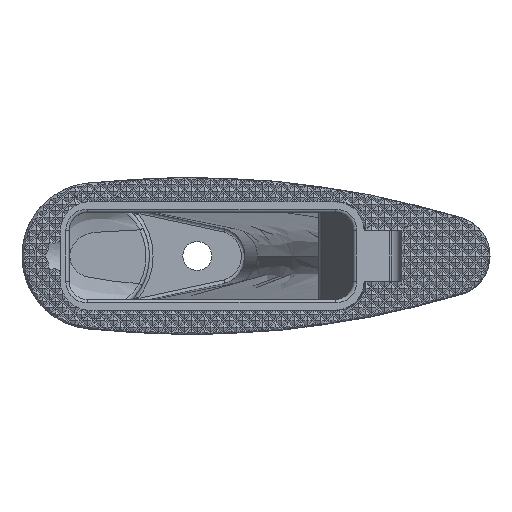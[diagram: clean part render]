
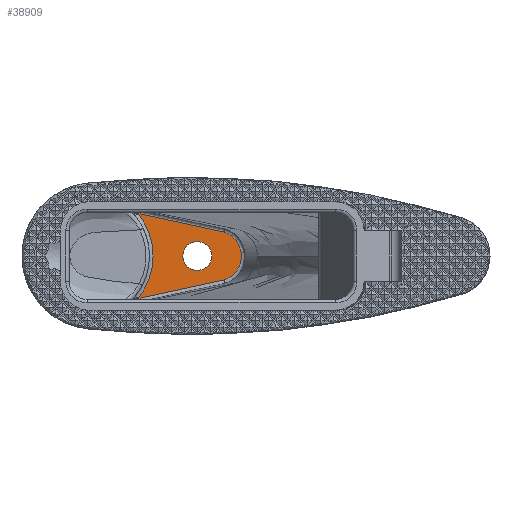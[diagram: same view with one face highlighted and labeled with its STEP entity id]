
A CAD part, left-side view. The second image highlights one B-rep face of the part: STEP entity #38909.
In plain terms, the highlighted planar face has unit normal (-1, 0, 0).
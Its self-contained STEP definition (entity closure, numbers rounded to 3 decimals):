
#926 = CIRCLE ( 'NONE', #54261, 4. ) ;
#2425 = FACE_BOUND ( 'NONE', #10219, .T. ) ;
#3760 = CARTESIAN_POINT ( 'NONE',  ( -210.6, -15.971, 6.591 ) ) ;
#4138 = CARTESIAN_POINT ( 'NONE',  ( -210.6, -20.515, 1.795 ) ) ;
#4658 = CARTESIAN_POINT ( 'NONE',  ( -210.6, 7.884, 11.758 ) ) ;
#5381 = VERTEX_POINT ( 'NONE', #7635 ) ;
#6216 = EDGE_CURVE ( 'NONE', #59459, #5381, #926, .T. ) ;
#7563 = B_SPLINE_CURVE_WITH_KNOTS ( 'NONE', 3,
 ( #16736, #67531, #17802, #61028, #34142, #17455, #34846 ),
 .UNSPECIFIED., .F., .F.,
 ( 4, 3, 4 ),
 ( 0., 0.011, 0.024 ),
 .UNSPECIFIED. ) ;
#7635 = CARTESIAN_POINT ( 'NONE',  ( -210.6, -8.516, 4. ) ) ;
#8342 = EDGE_CURVE ( 'NONE', #41749, #38159, #14809, .T. ) ;
#8493 = CARTESIAN_POINT ( 'NONE',  ( -210.6, -17.299, -6.008 ) ) ;
#9565 = CARTESIAN_POINT ( 'NONE',  ( -210.6, -20.74, 0.364 ) ) ;
#9740 = CARTESIAN_POINT ( 'NONE',  ( -210.6, 1.039, 10.275 ) ) ;
#9785 = CIRCLE ( 'NONE', #38876, 4. ) ;
#10219 = EDGE_LOOP ( 'NONE', ( #63972, #31793 ) ) ;
#11646 = ORIENTED_EDGE ( 'NONE', *, *, #71557, .T. ) ;
#12875 = CARTESIAN_POINT ( 'NONE',  ( -210.6, -16.648, -6.341 ) ) ;
#12945 = CARTESIAN_POINT ( 'NONE',  ( -210.6, -8.516, 0. ) ) ;
#13239 = CARTESIAN_POINT ( 'NONE',  ( -210.6, -16.314, -6.479 ) ) ;
#14061 = DIRECTION ( 'NONE',  ( -1., 0., 0. ) ) ;
#14809 = B_SPLINE_CURVE_WITH_KNOTS ( 'NONE', 3,
 ( #64927, #15202, #59492, #65276, #9740, #59859, #4658 ),
 .UNSPECIFIED., .F., .F.,
 ( 4, 3, 4 ),
 ( 0., 0.014, 0.024 ),
 .UNSPECIFIED. ) ;
#15202 = CARTESIAN_POINT ( 'NONE',  ( -210.6, -11.442, 7.573 ) ) ;
#15753 = CARTESIAN_POINT ( 'NONE',  ( -210.6, -20.599, -1.442 ) ) ;
#15930 = EDGE_LOOP ( 'NONE', ( #23929, #38214, #65621, #11646 ) ) ;
#16736 = CARTESIAN_POINT ( 'NONE',  ( -210.6, 7.884, -11.758 ) ) ;
#17455 = CARTESIAN_POINT ( 'NONE',  ( -210.6, -11.442, -7.573 ) ) ;
#17802 = CARTESIAN_POINT ( 'NONE',  ( -210.6, 1.039, -10.275 ) ) ;
#19174 = EDGE_CURVE ( 'NONE', #5381, #59459, #9785, .T. ) ;
#20528 = CARTESIAN_POINT ( 'NONE',  ( -210.6, -15.971, 6.591 ) ) ;
#21126 = DIRECTION ( 'NONE',  ( 1., 0., 0. ) ) ;
#23216 = CARTESIAN_POINT ( 'NONE',  ( -210.6, -15.971, -6.591 ) ) ;
#23788 = CARTESIAN_POINT ( 'NONE',  ( -210.6, -18.191, -5.392 ) ) ;
#23929 = ORIENTED_EDGE ( 'NONE', *, *, #8342, .T. ) ;
#24179 = DIRECTION ( 'NONE',  ( 0., 0., 1. ) ) ;
#25938 = CARTESIAN_POINT ( 'NONE',  ( -210.6, -18.49, 5.173 ) ) ;
#26308 = CARTESIAN_POINT ( 'NONE',  ( -210.6, -19.215, -4.361 ) ) ;
#26653 = CARTESIAN_POINT ( 'NONE',  ( -210.6, -20.74, -0.36 ) ) ;
#29328 = PLANE ( 'NONE',  #47952 ) ;
#29367 = VERTEX_POINT ( 'NONE', #23216 ) ;
#30736 = CARTESIAN_POINT ( 'NONE',  ( -210.6, -8.516, -4. ) ) ;
#31034 = CARTESIAN_POINT ( 'NONE',  ( -210.6, -20.292, 2.486 ) ) ;
#31381 = CARTESIAN_POINT ( 'NONE',  ( -210.6, -20.6, 1.437 ) ) ;
#31699 = AXIS2_PLACEMENT_3D ( 'NONE', #41950, #68092, #24179 ) ;
#31793 = ORIENTED_EDGE ( 'NONE', *, *, #19174, .T. ) ;
#31822 = VERTEX_POINT ( 'NONE', #70062 ) ;
#34142 = CARTESIAN_POINT ( 'NONE',  ( -210.6, -6.913, -8.553 ) ) ;
#34846 = CARTESIAN_POINT ( 'NONE',  ( -210.6, -15.971, -6.591 ) ) ;
#36461 = CARTESIAN_POINT ( 'NONE',  ( -210.6, -17.309, 6.036 ) ) ;
#37177 = CARTESIAN_POINT ( 'NONE',  ( -210.6, -19.828, 3.463 ) ) ;
#37899 = CARTESIAN_POINT ( 'NONE',  ( -210.6, -20.154, 2.819 ) ) ;
#38130 = EDGE_CURVE ( 'NONE', #38159, #31822, #67640, .T. ) ;
#38159 = VERTEX_POINT ( 'NONE', #71323 ) ;
#38214 = ORIENTED_EDGE ( 'NONE', *, *, #38130, .T. ) ;
#38876 = AXIS2_PLACEMENT_3D ( 'NONE', #12945, #50735, #51796 ) ;
#38909 = ADVANCED_FACE ( 'NONE', ( #2425, #46724 ), #29328, .T. ) ;
#40559 = DIRECTION ( 'NONE',  ( 0., 0., 1. ) ) ;
#41749 = VERTEX_POINT ( 'NONE', #20528 ) ;
#41950 = CARTESIAN_POINT ( 'NONE',  ( -210.6, 22.35, 0. ) ) ;
#42985 = CARTESIAN_POINT ( 'NONE',  ( -210.6, -20.294, -2.481 ) ) ;
#43343 = CARTESIAN_POINT ( 'NONE',  ( -210.6, -18.998, 4.661 ) ) ;
#46724 = FACE_OUTER_BOUND ( 'NONE', #15930, .T. ) ;
#47702 = CARTESIAN_POINT ( 'NONE',  ( -210.6, -20.712, 0.724 ) ) ;
#47952 = AXIS2_PLACEMENT_3D ( 'NONE', #63051, #14061, #40559 ) ;
#48020 = EDGE_CURVE ( 'NONE', #31822, #29367, #7563, .T. ) ;
#48064 = CARTESIAN_POINT ( 'NONE',  ( -210.6, -19.638, 3.775 ) ) ;
#48435 = CARTESIAN_POINT ( 'NONE',  ( -210.6, -16.666, 6.365 ) ) ;
#48781 = CARTESIAN_POINT ( 'NONE',  ( -210.6, -20.515, -1.793 ) ) ;
#49131 = B_SPLINE_CURVE_WITH_KNOTS ( 'NONE', 3,
 ( #58242, #13239, #12875, #8493, #51356, #23788, #68052, #53876, #26308, #70212, #59322, #64759, #42985, #48781, #15753, #65111, #26653, #9565, #47702, #31381, #4138, #31034, #37899, #37177, #48064, #43343, #25938, #36461, #48435, #3760 ),
 .UNSPECIFIED., .F., .F.,
 ( 4, 2, 2, 2, 2, 2, 2, 2, 2, 2, 2, 2, 2, 2, 4 ),
 ( 0.01, 0.012, 0.013, 0.014, 0.015, 0.016, 0.017, 0.018, 0.019, 0.02, 0.021, 0.022, 0.023, 0.026, 0.028 ),
 .UNSPECIFIED. ) ;
#50735 = DIRECTION ( 'NONE',  ( 1., 0., 0. ) ) ;
#51356 = CARTESIAN_POINT ( 'NONE',  ( -210.6, -17.608, -5.817 ) ) ;
#51796 = DIRECTION ( 'NONE',  ( 0., 0., 1. ) ) ;
#53812 = CARTESIAN_POINT ( 'NONE',  ( -210.6, -8.516, 0. ) ) ;
#53876 = CARTESIAN_POINT ( 'NONE',  ( -210.6, -18.978, -4.641 ) ) ;
#54261 = AXIS2_PLACEMENT_3D ( 'NONE', #53812, #21126, #59976 ) ;
#58242 = CARTESIAN_POINT ( 'NONE',  ( -210.6, -15.971, -6.591 ) ) ;
#59322 = CARTESIAN_POINT ( 'NONE',  ( -210.6, -19.825, -3.468 ) ) ;
#59459 = VERTEX_POINT ( 'NONE', #30736 ) ;
#59492 = CARTESIAN_POINT ( 'NONE',  ( -210.6, -6.913, 8.553 ) ) ;
#59859 = CARTESIAN_POINT ( 'NONE',  ( -210.6, 4.462, 11.016 ) ) ;
#59976 = DIRECTION ( 'NONE',  ( 0., 0., 1. ) ) ;
#61028 = CARTESIAN_POINT ( 'NONE',  ( -210.6, -2.383, -9.534 ) ) ;
#63051 = CARTESIAN_POINT ( 'NONE',  ( -210.6, 22.35, 0. ) ) ;
#63972 = ORIENTED_EDGE ( 'NONE', *, *, #6216, .T. ) ;
#64759 = CARTESIAN_POINT ( 'NONE',  ( -210.6, -20.153, -2.821 ) ) ;
#64927 = CARTESIAN_POINT ( 'NONE',  ( -210.6, -15.971, 6.591 ) ) ;
#65111 = CARTESIAN_POINT ( 'NONE',  ( -210.6, -20.712, -0.727 ) ) ;
#65276 = CARTESIAN_POINT ( 'NONE',  ( -210.6, -2.383, 9.534 ) ) ;
#65621 = ORIENTED_EDGE ( 'NONE', *, *, #48020, .T. ) ;
#67531 = CARTESIAN_POINT ( 'NONE',  ( -210.6, 4.462, -11.016 ) ) ;
#67640 = CIRCLE ( 'NONE', #31699, 18.641 ) ;
#68052 = CARTESIAN_POINT ( 'NONE',  ( -210.6, -18.465, -5.157 ) ) ;
#68092 = DIRECTION ( 'NONE',  ( 1., 0., 0. ) ) ;
#70062 = CARTESIAN_POINT ( 'NONE',  ( -210.6, 7.884, -11.758 ) ) ;
#70212 = CARTESIAN_POINT ( 'NONE',  ( -210.6, -19.638, -3.776 ) ) ;
#71323 = CARTESIAN_POINT ( 'NONE',  ( -210.6, 7.884, 11.758 ) ) ;
#71557 = EDGE_CURVE ( 'NONE', #29367, #41749, #49131, .T. ) ;
